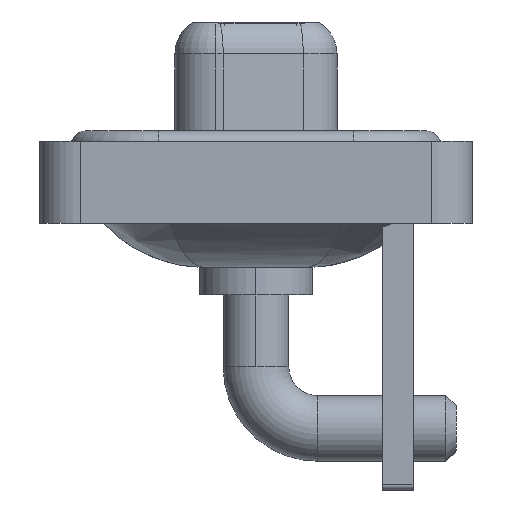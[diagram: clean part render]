
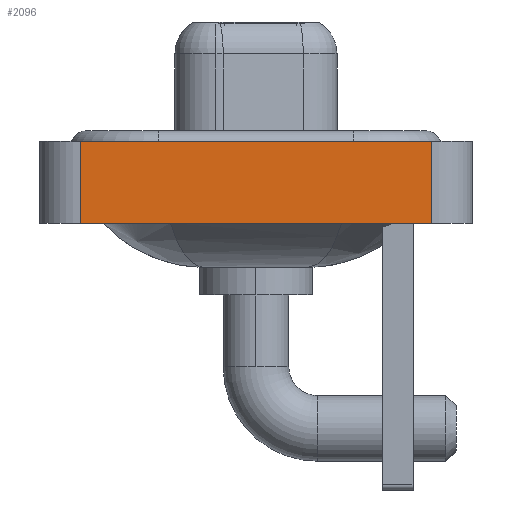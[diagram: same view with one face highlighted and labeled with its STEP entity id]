
A CAD part, left-side view. The second image highlights one B-rep face of the part: STEP entity #2096.
In plain terms, the highlighted planar face has unit normal (-1, 0, 0).
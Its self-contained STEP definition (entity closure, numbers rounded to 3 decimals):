
#384 = DIRECTION ( 'NONE',  ( 0., 0., 1. ) ) ;
#775 = ORIENTED_EDGE ( 'NONE', *, *, #14826, .F. ) ;
#1814 = CARTESIAN_POINT ( 'NONE',  ( -7.3, 8.55, 0.4 ) ) ;
#2096 = ADVANCED_FACE ( 'NONE', ( #5616 ), #16119, .T. ) ;
#2656 = DIRECTION ( 'NONE',  ( 0., 0., 1. ) ) ;
#2978 = EDGE_CURVE ( 'NONE', #4182, #9745, #14250, .T. ) ;
#3174 = ORIENTED_EDGE ( 'NONE', *, *, #2978, .T. ) ;
#3431 = CARTESIAN_POINT ( 'NONE',  ( -7.3, 8.55, -3.6 ) ) ;
#3937 = CARTESIAN_POINT ( 'NONE',  ( -7.3, -8.55, -3.6 ) ) ;
#4182 = VERTEX_POINT ( 'NONE', #3431 ) ;
#5090 = DIRECTION ( 'NONE',  ( 0., -1., 0. ) ) ;
#5616 = FACE_OUTER_BOUND ( 'NONE', #15165, .T. ) ;
#5913 = CARTESIAN_POINT ( 'NONE',  ( -7.3, -8.55, -3.6 ) ) ;
#6534 = CARTESIAN_POINT ( 'NONE',  ( -7.3, -8.55, 0.4 ) ) ;
#6904 = VERTEX_POINT ( 'NONE', #11926 ) ;
#7086 = ORIENTED_EDGE ( 'NONE', *, *, #14070, .T. ) ;
#8727 = LINE ( 'NONE', #10179, #13742 ) ;
#8981 = CARTESIAN_POINT ( 'NONE',  ( -7.3, -8.55, -3.6 ) ) ;
#9591 = VECTOR ( 'NONE', #5090, 1000. ) ;
#9745 = VERTEX_POINT ( 'NONE', #5913 ) ;
#10101 = VECTOR ( 'NONE', #2656, 1000. ) ;
#10179 = CARTESIAN_POINT ( 'NONE',  ( -7.3, 8.55, -3.6 ) ) ;
#11106 = ORIENTED_EDGE ( 'NONE', *, *, #11542, .F. ) ;
#11542 = EDGE_CURVE ( 'NONE', #4182, #12167, #8727, .T. ) ;
#11926 = CARTESIAN_POINT ( 'NONE',  ( -7.3, -8.55, 0.4 ) ) ;
#12167 = VERTEX_POINT ( 'NONE', #1814 ) ;
#12881 = DIRECTION ( 'NONE',  ( 0., -1., 0. ) ) ;
#13067 = LINE ( 'NONE', #3937, #10101 ) ;
#13134 = VECTOR ( 'NONE', #12881, 1000. ) ;
#13742 = VECTOR ( 'NONE', #13909, 1000. ) ;
#13909 = DIRECTION ( 'NONE',  ( 0., 0., 1. ) ) ;
#14070 = EDGE_CURVE ( 'NONE', #9745, #6904, #13067, .T. ) ;
#14213 = LINE ( 'NONE', #6534, #9591 ) ;
#14250 = LINE ( 'NONE', #8981, #13134 ) ;
#14826 = EDGE_CURVE ( 'NONE', #12167, #6904, #14213, .T. ) ;
#14844 = DIRECTION ( 'NONE',  ( -1., 0., 0. ) ) ;
#15165 = EDGE_LOOP ( 'NONE', ( #7086, #775, #11106, #3174 ) ) ;
#16029 = CARTESIAN_POINT ( 'NONE',  ( -7.3, -8.55, -3.6 ) ) ;
#16119 = PLANE ( 'NONE',  #16678 ) ;
#16678 = AXIS2_PLACEMENT_3D ( 'NONE', #16029, #14844, #384 ) ;
